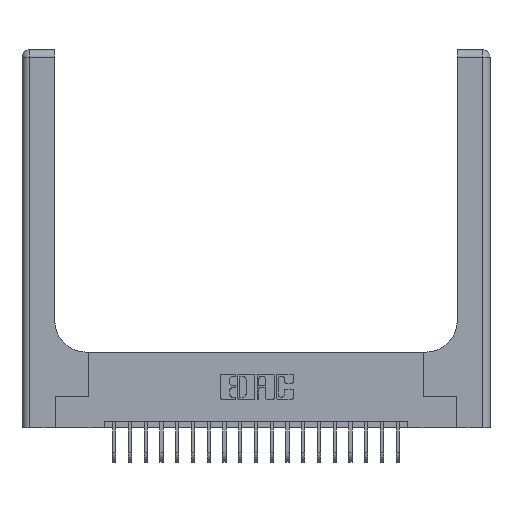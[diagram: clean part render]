
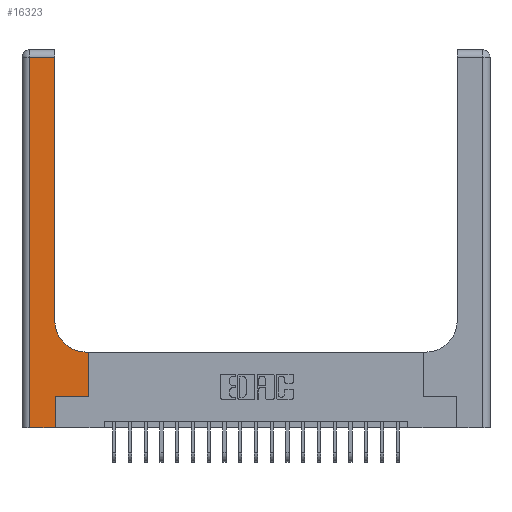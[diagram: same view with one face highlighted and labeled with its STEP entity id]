
A CAD part, top view. The second image highlights one B-rep face of the part: STEP entity #16323.
In plain terms, the highlighted planar face has unit normal (0, 0, 1).
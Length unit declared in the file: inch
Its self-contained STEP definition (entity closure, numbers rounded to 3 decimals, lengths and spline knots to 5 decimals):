
#833 = CARTESIAN_POINT ( 'NONE',  ( 0.51, 0.85, 0.37 ) ) ;
#1018 = CARTESIAN_POINT ( 'NONE',  ( 0.51, 0.6, 0.37 ) ) ;
#1258 = VERTEX_POINT ( 'NONE', #2098 ) ;
#1887 = CARTESIAN_POINT ( 'NONE',  ( 0.26, 2.94, 0.37 ) ) ;
#2098 = CARTESIAN_POINT ( 'NONE',  ( 0.528, 0.6, 0.37 ) ) ;
#2651 = VECTOR ( 'NONE', #12429, 39.37008 ) ;
#2784 = CARTESIAN_POINT ( 'NONE',  ( 0.265, 0.25, 0.37 ) ) ;
#2984 = VERTEX_POINT ( 'NONE', #1887 ) ;
#3873 = DIRECTION ( 'NONE',  ( 0., 0., -1. ) ) ;
#3976 = VECTOR ( 'NONE', #4556, 39.37008 ) ;
#4073 = DIRECTION ( 'NONE',  ( -1., 0., 0. ) ) ;
#4180 = PLANE ( 'NONE',  #11777 ) ;
#4556 = DIRECTION ( 'NONE',  ( 0., -1., 0. ) ) ;
#4591 = CARTESIAN_POINT ( 'NONE',  ( 0.26, 0.6, 0.37 ) ) ;
#5633 = EDGE_LOOP ( 'NONE', ( #10528, #16705, #6118, #12672, #5897, #13244, #6105, #12836, #10331 ) ) ;
#5787 = LINE ( 'NONE', #12147, #10023 ) ;
#5897 = ORIENTED_EDGE ( 'NONE', *, *, #12268, .T. ) ;
#6105 = ORIENTED_EDGE ( 'NONE', *, *, #13515, .T. ) ;
#6118 = ORIENTED_EDGE ( 'NONE', *, *, #9898, .T. ) ;
#6245 = EDGE_CURVE ( 'NONE', #15588, #2984, #13550, .T. ) ;
#6250 = EDGE_CURVE ( 'NONE', #9230, #18287, #13747, .T. ) ;
#6750 = EDGE_CURVE ( 'NONE', #2984, #9063, #17461, .T. ) ;
#7381 = DIRECTION ( 'NONE',  ( 0., 1., 0. ) ) ;
#7770 = CARTESIAN_POINT ( 'NONE',  ( 0.06, 3., 0.37 ) ) ;
#8745 = CARTESIAN_POINT ( 'NONE',  ( 0.265, 0.25, 0.37 ) ) ;
#8861 = CARTESIAN_POINT ( 'NONE',  ( 0.06, 0., 0.37 ) ) ;
#8950 = DIRECTION ( 'NONE',  ( 1., 0., 0. ) ) ;
#9063 = VERTEX_POINT ( 'NONE', #17409 ) ;
#9113 = CARTESIAN_POINT ( 'NONE',  ( 0., 0., 0.37 ) ) ;
#9230 = VERTEX_POINT ( 'NONE', #8745 ) ;
#9443 = DIRECTION ( 'NONE',  ( -1., 0., 0. ) ) ;
#9898 = EDGE_CURVE ( 'NONE', #9063, #16324, #12897, .T. ) ;
#9920 = DIRECTION ( 'NONE',  ( 1., 0., 0. ) ) ;
#10023 = VECTOR ( 'NONE', #18503, 39.37008 ) ;
#10204 = EDGE_CURVE ( 'NONE', #16324, #11796, #18595, .T. ) ;
#10331 = ORIENTED_EDGE ( 'NONE', *, *, #19552, .T. ) ;
#10528 = ORIENTED_EDGE ( 'NONE', *, *, #6245, .T. ) ;
#11309 = VECTOR ( 'NONE', #7381, 39.37008 ) ;
#11777 = AXIS2_PLACEMENT_3D ( 'NONE', #14914, #3873, #4073 ) ;
#11796 = VERTEX_POINT ( 'NONE', #16644 ) ;
#12147 = CARTESIAN_POINT ( 'NONE',  ( 0.528, 0.25, 0.37 ) ) ;
#12268 = EDGE_CURVE ( 'NONE', #11796, #9230, #17313, .T. ) ;
#12429 = DIRECTION ( 'NONE',  ( 0., 1., 0. ) ) ;
#12672 = ORIENTED_EDGE ( 'NONE', *, *, #10204, .T. ) ;
#12705 = VECTOR ( 'NONE', #16695, 39.37008 ) ;
#12836 = ORIENTED_EDGE ( 'NONE', *, *, #13863, .T. ) ;
#12897 = LINE ( 'NONE', #7770, #3976 ) ;
#13028 = VERTEX_POINT ( 'NONE', #1018 ) ;
#13244 = ORIENTED_EDGE ( 'NONE', *, *, #6250, .T. ) ;
#13303 = VECTOR ( 'NONE', #8950, 39.37008 ) ;
#13487 = AXIS2_PLACEMENT_3D ( 'NONE', #833, #17837, #9920 ) ;
#13515 = EDGE_CURVE ( 'NONE', #18287, #1258, #5787, .T. ) ;
#13550 = LINE ( 'NONE', #15208, #11309 ) ;
#13747 = LINE ( 'NONE', #2784, #13303 ) ;
#13863 = EDGE_CURVE ( 'NONE', #1258, #13028, #17394, .T. ) ;
#14471 = CIRCLE ( 'NONE', #13487, 0.25 ) ;
#14914 = CARTESIAN_POINT ( 'NONE',  ( 0., 3., 0.37 ) ) ;
#15208 = CARTESIAN_POINT ( 'NONE',  ( 0.26, 3., 0.37 ) ) ;
#15261 = DIRECTION ( 'NONE',  ( 1., 0., 0. ) ) ;
#15584 = CARTESIAN_POINT ( 'NONE',  ( 0., 2.94, 0.37 ) ) ;
#15588 = VERTEX_POINT ( 'NONE', #15779 ) ;
#15637 = VECTOR ( 'NONE', #15261, 39.37008 ) ;
#15779 = CARTESIAN_POINT ( 'NONE',  ( 0.26, 0.85, 0.37 ) ) ;
#15862 = CARTESIAN_POINT ( 'NONE',  ( 0.265, 0., 0.37 ) ) ;
#16323 = ADVANCED_FACE ( 'NONE', ( #16477 ), #4180, .F. ) ;
#16324 = VERTEX_POINT ( 'NONE', #8861 ) ;
#16477 = FACE_OUTER_BOUND ( 'NONE', #5633, .T. ) ;
#16644 = CARTESIAN_POINT ( 'NONE',  ( 0.265, 0., 0.37 ) ) ;
#16695 = DIRECTION ( 'NONE',  ( -1., 0., 0. ) ) ;
#16705 = ORIENTED_EDGE ( 'NONE', *, *, #6750, .T. ) ;
#17313 = LINE ( 'NONE', #15862, #2651 ) ;
#17394 = LINE ( 'NONE', #4591, #12705 ) ;
#17409 = CARTESIAN_POINT ( 'NONE',  ( 0.06, 2.94, 0.37 ) ) ;
#17461 = LINE ( 'NONE', #15584, #18045 ) ;
#17837 = DIRECTION ( 'NONE',  ( 0., 0., -1. ) ) ;
#18045 = VECTOR ( 'NONE', #9443, 39.37008 ) ;
#18287 = VERTEX_POINT ( 'NONE', #20157 ) ;
#18503 = DIRECTION ( 'NONE',  ( 0., 1., 0. ) ) ;
#18595 = LINE ( 'NONE', #9113, #15637 ) ;
#19552 = EDGE_CURVE ( 'NONE', #13028, #15588, #14471, .T. ) ;
#20157 = CARTESIAN_POINT ( 'NONE',  ( 0.528, 0.25, 0.37 ) ) ;
